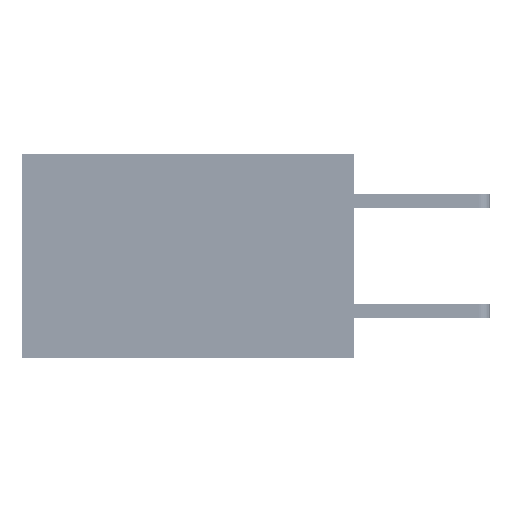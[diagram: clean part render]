
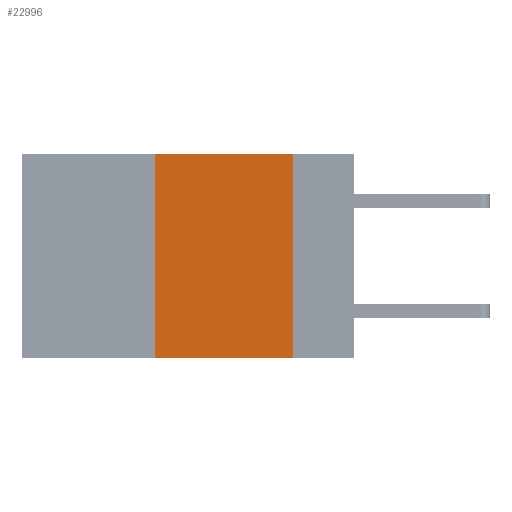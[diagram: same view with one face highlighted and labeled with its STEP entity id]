
A CAD part, left-side view. The second image highlights one B-rep face of the part: STEP entity #22996.
In plain terms, the highlighted planar face has unit normal (-1, 0, 0).
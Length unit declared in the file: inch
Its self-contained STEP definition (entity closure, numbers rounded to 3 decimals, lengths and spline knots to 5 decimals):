
#1098 = VERTEX_POINT ( 'NONE', #13839 ) ;
#2439 = VERTEX_POINT ( 'NONE', #27927 ) ;
#4700 = DIRECTION ( 'NONE',  ( 1., 0., 0. ) ) ;
#5579 = EDGE_CURVE ( 'NONE', #2439, #34953, #30660, .T. ) ;
#7043 = AXIS2_PLACEMENT_3D ( 'NONE', #24478, #4700, #9114 ) ;
#7194 = DIRECTION ( 'NONE',  ( 0., 0., -1. ) ) ;
#7718 = EDGE_CURVE ( 'NONE', #9860, #1098, #45499, .T. ) ;
#8639 = ORIENTED_EDGE ( 'NONE', *, *, #47228, .T. ) ;
#9114 = DIRECTION ( 'NONE',  ( 0., 0., -1. ) ) ;
#9860 = VERTEX_POINT ( 'NONE', #28171 ) ;
#11301 = VECTOR ( 'NONE', #21034, 39.37008 ) ;
#11748 = ORIENTED_EDGE ( 'NONE', *, *, #7718, .F. ) ;
#12600 = VECTOR ( 'NONE', #17132, 39.37008 ) ;
#13839 = CARTESIAN_POINT ( 'NONE',  ( 0., 0.11, -0.37 ) ) ;
#14884 = EDGE_LOOP ( 'NONE', ( #11748, #25789, #45064, #8639 ) ) ;
#17132 = DIRECTION ( 'NONE',  ( 0., 0., 1. ) ) ;
#18551 = CARTESIAN_POINT ( 'NONE',  ( 0., 0.11, 0. ) ) ;
#21034 = DIRECTION ( 'NONE',  ( 0., -1., 0. ) ) ;
#22996 = ADVANCED_FACE ( 'NONE', ( #42695 ), #35723, .F. ) ;
#24478 = CARTESIAN_POINT ( 'NONE',  ( 0., 0.6, 0. ) ) ;
#24545 = CARTESIAN_POINT ( 'NONE',  ( 0., 0.6, 0. ) ) ;
#25786 = LINE ( 'NONE', #36625, #11301 ) ;
#25789 = ORIENTED_EDGE ( 'NONE', *, *, #28352, .F. ) ;
#27927 = CARTESIAN_POINT ( 'NONE',  ( 0., 0.36, -0.37 ) ) ;
#28171 = CARTESIAN_POINT ( 'NONE',  ( 0., 0.11, 0. ) ) ;
#28352 = EDGE_CURVE ( 'NONE', #34953, #9860, #42251, .T. ) ;
#30430 = CARTESIAN_POINT ( 'NONE',  ( 0., 0.36, 0. ) ) ;
#30660 = LINE ( 'NONE', #36273, #12600 ) ;
#33758 = VECTOR ( 'NONE', #36452, 39.37008 ) ;
#34953 = VERTEX_POINT ( 'NONE', #30430 ) ;
#35723 = PLANE ( 'NONE',  #7043 ) ;
#36273 = CARTESIAN_POINT ( 'NONE',  ( 0., 0.36, 0. ) ) ;
#36452 = DIRECTION ( 'NONE',  ( 0., -1., 0. ) ) ;
#36625 = CARTESIAN_POINT ( 'NONE',  ( 0., 0.6, -0.37 ) ) ;
#42251 = LINE ( 'NONE', #24545, #33758 ) ;
#42695 = FACE_OUTER_BOUND ( 'NONE', #14884, .T. ) ;
#44913 = VECTOR ( 'NONE', #7194, 39.37008 ) ;
#45064 = ORIENTED_EDGE ( 'NONE', *, *, #5579, .F. ) ;
#45499 = LINE ( 'NONE', #18551, #44913 ) ;
#47228 = EDGE_CURVE ( 'NONE', #2439, #1098, #25786, .T. ) ;
